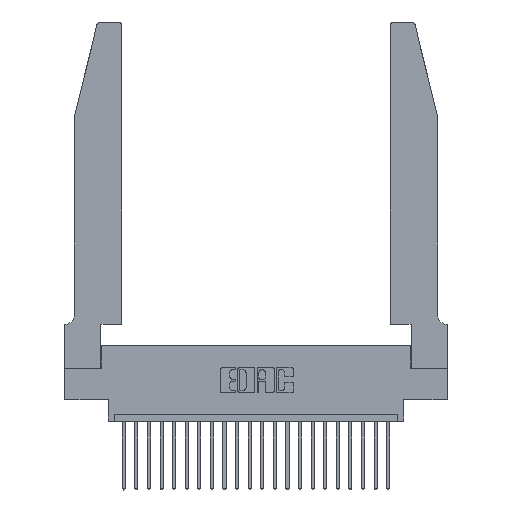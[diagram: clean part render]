
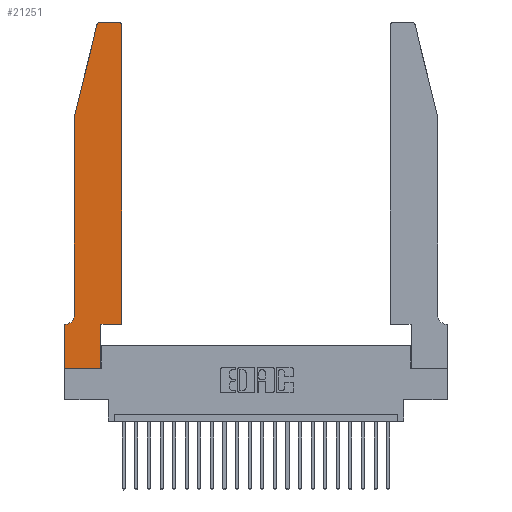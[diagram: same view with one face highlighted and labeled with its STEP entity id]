
A CAD part, top view. The second image highlights one B-rep face of the part: STEP entity #21251.
In plain terms, the highlighted planar face has unit normal (0, 0, 1).
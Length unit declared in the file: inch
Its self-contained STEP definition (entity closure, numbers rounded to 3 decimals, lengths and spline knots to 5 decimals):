
#561 = VECTOR ( 'NONE', #2851, 39.37008 ) ;
#818 = DIRECTION ( 'NONE',  ( -1., 0., 0. ) ) ;
#875 = PLANE ( 'NONE',  #2946 ) ;
#922 = VECTOR ( 'NONE', #21146, 39.37008 ) ;
#951 = CARTESIAN_POINT ( 'NONE',  ( 0.284, 2.72, 0.37 ) ) ;
#980 = CARTESIAN_POINT ( 'NONE',  ( 0.0755, 2., 0.37 ) ) ;
#1284 = VERTEX_POINT ( 'NONE', #8425 ) ;
#1343 = EDGE_LOOP ( 'NONE', ( #22157, #12127, #10126, #18571, #16006, #3746, #15037, #8432, #13112, #10556, #4398, #22718 ) ) ;
#1498 = VERTEX_POINT ( 'NONE', #6287 ) ;
#1759 = CIRCLE ( 'NONE', #4631, 0.03 ) ;
#1848 = LINE ( 'NONE', #9418, #11417 ) ;
#2017 = DIRECTION ( 'NONE',  ( 0., 0., 1. ) ) ;
#2116 = DIRECTION ( 'NONE',  ( 0., 1., 0. ) ) ;
#2393 = EDGE_CURVE ( 'NONE', #1498, #1284, #22871, .T. ) ;
#2420 = CARTESIAN_POINT ( 'NONE',  ( 0.2865, 0.35, 0.37 ) ) ;
#2446 = VECTOR ( 'NONE', #12470, 39.37008 ) ;
#2723 = EDGE_CURVE ( 'NONE', #9472, #17674, #1848, .T. ) ;
#2745 = DIRECTION ( 'NONE',  ( 0., -1., 0. ) ) ;
#2765 = EDGE_CURVE ( 'NONE', #14096, #13410, #21069, .T. ) ;
#2851 = DIRECTION ( 'NONE',  ( -0.239, -0.971, 0. ) ) ;
#2946 = AXIS2_PLACEMENT_3D ( 'NONE', #10598, #14383, #18378 ) ;
#3086 = VECTOR ( 'NONE', #2745, 39.37008 ) ;
#3746 = ORIENTED_EDGE ( 'NONE', *, *, #2393, .T. ) ;
#3925 = DIRECTION ( 'NONE',  ( 0., 1., 0. ) ) ;
#4171 = VERTEX_POINT ( 'NONE', #13539 ) ;
#4241 = CARTESIAN_POINT ( 'NONE',  ( 0.0055, 0.42, 0.37 ) ) ;
#4398 = ORIENTED_EDGE ( 'NONE', *, *, #2723, .T. ) ;
#4516 = VECTOR ( 'NONE', #19345, 39.37008 ) ;
#4631 = AXIS2_PLACEMENT_3D ( 'NONE', #21739, #2017, #7036 ) ;
#6108 = DIRECTION ( 'NONE',  ( -1., 0., 0. ) ) ;
#6242 = CARTESIAN_POINT ( 'NONE',  ( 0., 0., 0.37 ) ) ;
#6287 = CARTESIAN_POINT ( 'NONE',  ( 0.0055, 0.35, 0.37 ) ) ;
#6452 = CARTESIAN_POINT ( 'NONE',  ( 0.0755, 0.42, 0.37 ) ) ;
#6490 = DIRECTION ( 'NONE',  ( 0., 0., 1. ) ) ;
#7030 = AXIS2_PLACEMENT_3D ( 'NONE', #4241, #15438, #6108 ) ;
#7036 = DIRECTION ( 'NONE',  ( 1., 0., 0. ) ) ;
#7238 = EDGE_CURVE ( 'NONE', #4171, #8857, #13403, .T. ) ;
#8425 = CARTESIAN_POINT ( 'NONE',  ( 0., 0.35, 0.37 ) ) ;
#8432 = ORIENTED_EDGE ( 'NONE', *, *, #10609, .T. ) ;
#8564 = CARTESIAN_POINT ( 'NONE',  ( 0.284, 2.75, 0.37 ) ) ;
#8857 = VERTEX_POINT ( 'NONE', #8564 ) ;
#9396 = LINE ( 'NONE', #6242, #4516 ) ;
#9418 = CARTESIAN_POINT ( 'NONE',  ( 0.4505, 0.35, 0.37 ) ) ;
#9472 = VERTEX_POINT ( 'NONE', #12869 ) ;
#10090 = VECTOR ( 'NONE', #10397, 39.37008 ) ;
#10126 = ORIENTED_EDGE ( 'NONE', *, *, #18072, .T. ) ;
#10150 = CARTESIAN_POINT ( 'NONE',  ( 0.2605, 2.75, 0.37 ) ) ;
#10236 = CARTESIAN_POINT ( 'NONE',  ( 0., 0., 0.37 ) ) ;
#10397 = DIRECTION ( 'NONE',  ( 0., -1., 0. ) ) ;
#10491 = LINE ( 'NONE', #13823, #922 ) ;
#10556 = ORIENTED_EDGE ( 'NONE', *, *, #17061, .T. ) ;
#10598 = CARTESIAN_POINT ( 'NONE',  ( 0., 0.35, 0.37 ) ) ;
#10609 = EDGE_CURVE ( 'NONE', #18037, #14096, #9396, .T. ) ;
#10614 = LINE ( 'NONE', #13895, #3086 ) ;
#10808 = EDGE_CURVE ( 'NONE', #8857, #22053, #17915, .T. ) ;
#11417 = VECTOR ( 'NONE', #3925, 39.37008 ) ;
#11754 = FACE_OUTER_BOUND ( 'NONE', #1343, .T. ) ;
#12015 = CIRCLE ( 'NONE', #7030, 0.07 ) ;
#12127 = ORIENTED_EDGE ( 'NONE', *, *, #10808, .T. ) ;
#12470 = DIRECTION ( 'NONE',  ( -1., 0., 0. ) ) ;
#12654 = AXIS2_PLACEMENT_3D ( 'NONE', #951, #6490, #19689 ) ;
#12869 = CARTESIAN_POINT ( 'NONE',  ( 0.4505, 0.35, 0.37 ) ) ;
#13112 = ORIENTED_EDGE ( 'NONE', *, *, #2765, .T. ) ;
#13248 = CARTESIAN_POINT ( 'NONE',  ( 0.4505, 2.72, 0.37 ) ) ;
#13255 = VERTEX_POINT ( 'NONE', #6452 ) ;
#13403 = LINE ( 'NONE', #10150, #23951 ) ;
#13410 = VERTEX_POINT ( 'NONE', #2420 ) ;
#13539 = CARTESIAN_POINT ( 'NONE',  ( 0.4205, 2.75, 0.37 ) ) ;
#13823 = CARTESIAN_POINT ( 'NONE',  ( 0.4505, 0.35, 0.37 ) ) ;
#13895 = CARTESIAN_POINT ( 'NONE',  ( 0.0755, 2., 0.37 ) ) ;
#14096 = VERTEX_POINT ( 'NONE', #17844 ) ;
#14383 = DIRECTION ( 'NONE',  ( 0., 0., 1. ) ) ;
#15037 = ORIENTED_EDGE ( 'NONE', *, *, #23482, .T. ) ;
#15438 = DIRECTION ( 'NONE',  ( 0., 0., -1. ) ) ;
#15880 = CARTESIAN_POINT ( 'NONE',  ( 0.0755, 2., 0.37 ) ) ;
#16006 = ORIENTED_EDGE ( 'NONE', *, *, #22170, .T. ) ;
#16103 = VECTOR ( 'NONE', #2116, 39.37008 ) ;
#16450 = EDGE_CURVE ( 'NONE', #19464, #13255, #10614, .T. ) ;
#17061 = EDGE_CURVE ( 'NONE', #13410, #9472, #10491, .T. ) ;
#17365 = EDGE_CURVE ( 'NONE', #17674, #4171, #1759, .T. ) ;
#17674 = VERTEX_POINT ( 'NONE', #13248 ) ;
#17844 = CARTESIAN_POINT ( 'NONE',  ( 0.2865, 0., 0.37 ) ) ;
#17847 = CARTESIAN_POINT ( 'NONE',  ( 0., 0., 0.37 ) ) ;
#17915 = CIRCLE ( 'NONE', #12654, 0.03 ) ;
#18037 = VERTEX_POINT ( 'NONE', #10236 ) ;
#18072 = EDGE_CURVE ( 'NONE', #22053, #19464, #20653, .T. ) ;
#18378 = DIRECTION ( 'NONE',  ( 1., 0., 0. ) ) ;
#18571 = ORIENTED_EDGE ( 'NONE', *, *, #16450, .T. ) ;
#19345 = DIRECTION ( 'NONE',  ( 1., 0., 0. ) ) ;
#19464 = VERTEX_POINT ( 'NONE', #15880 ) ;
#19689 = DIRECTION ( 'NONE',  ( 1., 0., 0. ) ) ;
#20046 = LINE ( 'NONE', #17847, #10090 ) ;
#20078 = CARTESIAN_POINT ( 'NONE',  ( 0.2865, 0.35, 0.37 ) ) ;
#20523 = CARTESIAN_POINT ( 'NONE',  ( 0.25487, 2.72718, 0.37 ) ) ;
#20653 = LINE ( 'NONE', #980, #561 ) ;
#21069 = LINE ( 'NONE', #20078, #16103 ) ;
#21146 = DIRECTION ( 'NONE',  ( 1., 0., 0. ) ) ;
#21251 = ADVANCED_FACE ( 'NONE', ( #11754 ), #875, .T. ) ;
#21694 = CARTESIAN_POINT ( 'NONE',  ( 0.0755, 0.35, 0.37 ) ) ;
#21739 = CARTESIAN_POINT ( 'NONE',  ( 0.4205, 2.72, 0.37 ) ) ;
#22053 = VERTEX_POINT ( 'NONE', #20523 ) ;
#22157 = ORIENTED_EDGE ( 'NONE', *, *, #7238, .T. ) ;
#22170 = EDGE_CURVE ( 'NONE', #13255, #1498, #12015, .T. ) ;
#22718 = ORIENTED_EDGE ( 'NONE', *, *, #17365, .T. ) ;
#22871 = LINE ( 'NONE', #21694, #2446 ) ;
#23482 = EDGE_CURVE ( 'NONE', #1284, #18037, #20046, .T. ) ;
#23951 = VECTOR ( 'NONE', #818, 39.37008 ) ;
